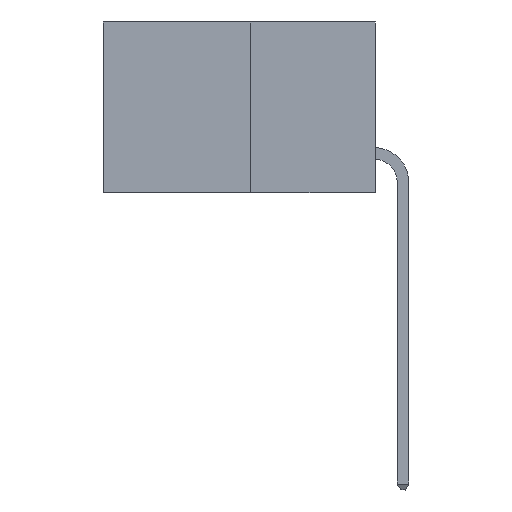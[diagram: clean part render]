
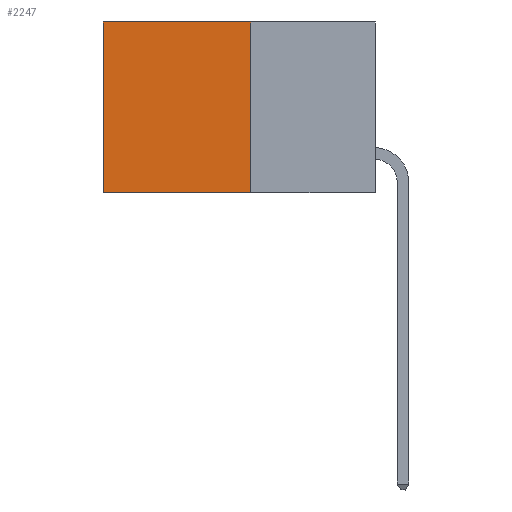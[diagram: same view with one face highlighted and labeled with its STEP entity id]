
A CAD part, left-side view. The second image highlights one B-rep face of the part: STEP entity #2247.
In plain terms, the highlighted planar face has unit normal (-1, 0, 0).
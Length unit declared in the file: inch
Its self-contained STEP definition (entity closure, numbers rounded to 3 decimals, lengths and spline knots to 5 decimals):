
#27 = LINE ( 'NONE', #1770, #15260 ) ;
#1605 = VERTEX_POINT ( 'NONE', #11497 ) ;
#1770 = CARTESIAN_POINT ( 'NONE',  ( 0.277, 0.27, -0.37 ) ) ;
#1911 = CARTESIAN_POINT ( 'NONE',  ( 0.277, 0.59, 0. ) ) ;
#2005 = DIRECTION ( 'NONE',  ( 0., 0., -1. ) ) ;
#2247 = ADVANCED_FACE ( 'NONE', ( #11431 ), #10173, .F. ) ;
#2573 = DIRECTION ( 'NONE',  ( 0., 0., -1. ) ) ;
#2735 = EDGE_LOOP ( 'NONE', ( #16464, #13527, #13225, #21986 ) ) ;
#3115 = DIRECTION ( 'NONE',  ( 0., 0., -1. ) ) ;
#4376 = CARTESIAN_POINT ( 'NONE',  ( 0.277, 0.27, -0.37 ) ) ;
#4438 = EDGE_CURVE ( 'NONE', #7517, #18368, #27, .T. ) ;
#5693 = CARTESIAN_POINT ( 'NONE',  ( 0.277, 0.59, -0.37 ) ) ;
#5854 = CARTESIAN_POINT ( 'NONE',  ( 0.277, 0.27, 0. ) ) ;
#7517 = VERTEX_POINT ( 'NONE', #23209 ) ;
#7712 = DIRECTION ( 'NONE',  ( 0., 1., 0. ) ) ;
#7786 = DIRECTION ( 'NONE',  ( 0., 1., 0. ) ) ;
#8207 = VERTEX_POINT ( 'NONE', #1911 ) ;
#9749 = VECTOR ( 'NONE', #2005, 39.37008 ) ;
#10173 = PLANE ( 'NONE',  #12320 ) ;
#11431 = FACE_OUTER_BOUND ( 'NONE', #2735, .T. ) ;
#11497 = CARTESIAN_POINT ( 'NONE',  ( 0.277, 0.59, -0.37 ) ) ;
#12156 = CARTESIAN_POINT ( 'NONE',  ( 0.277, 0.27, -0.37 ) ) ;
#12320 = AXIS2_PLACEMENT_3D ( 'NONE', #4376, #16876, #2573 ) ;
#13225 = ORIENTED_EDGE ( 'NONE', *, *, #4438, .F. ) ;
#13493 = VECTOR ( 'NONE', #7712, 39.37008 ) ;
#13527 = ORIENTED_EDGE ( 'NONE', *, *, #16930, .F. ) ;
#14614 = LINE ( 'NONE', #5693, #9749 ) ;
#15260 = VECTOR ( 'NONE', #3115, 39.37008 ) ;
#16464 = ORIENTED_EDGE ( 'NONE', *, *, #21161, .T. ) ;
#16876 = DIRECTION ( 'NONE',  ( 1., 0., 0. ) ) ;
#16930 = EDGE_CURVE ( 'NONE', #18368, #1605, #22755, .T. ) ;
#18287 = LINE ( 'NONE', #5854, #13493 ) ;
#18368 = VERTEX_POINT ( 'NONE', #12156 ) ;
#18698 = CARTESIAN_POINT ( 'NONE',  ( 0.277, 0.27, -0.37 ) ) ;
#21161 = EDGE_CURVE ( 'NONE', #8207, #1605, #14614, .T. ) ;
#21218 = EDGE_CURVE ( 'NONE', #7517, #8207, #18287, .T. ) ;
#21986 = ORIENTED_EDGE ( 'NONE', *, *, #21218, .T. ) ;
#22755 = LINE ( 'NONE', #18698, #23318 ) ;
#23209 = CARTESIAN_POINT ( 'NONE',  ( 0.277, 0.27, 0. ) ) ;
#23318 = VECTOR ( 'NONE', #7786, 39.37008 ) ;
